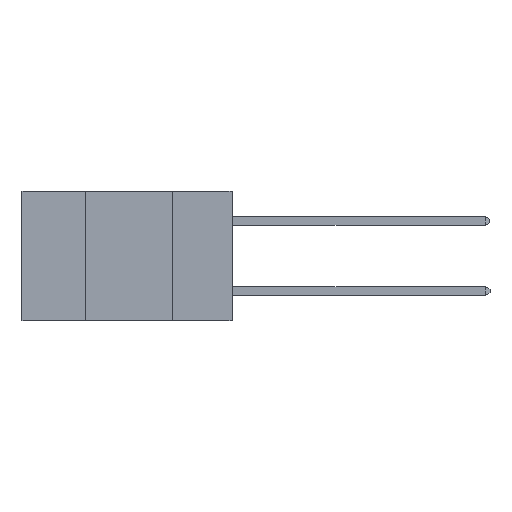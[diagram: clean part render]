
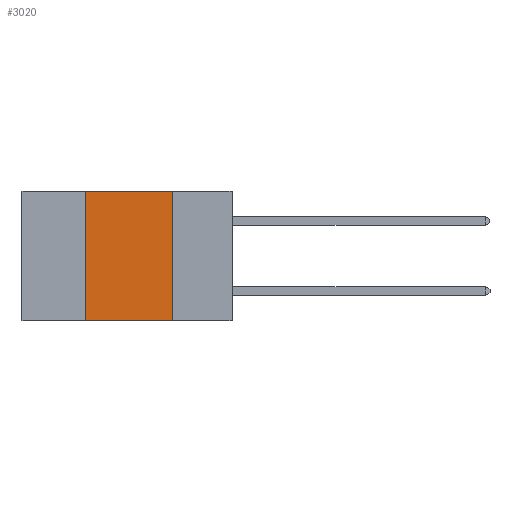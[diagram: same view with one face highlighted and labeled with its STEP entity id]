
A CAD part, left-side view. The second image highlights one B-rep face of the part: STEP entity #3020.
In plain terms, the highlighted planar face has unit normal (-1, 0, 0).
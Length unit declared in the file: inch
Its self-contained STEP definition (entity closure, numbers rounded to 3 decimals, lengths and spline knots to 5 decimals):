
#36 = DIRECTION ( 'NONE',  ( 0., 0., 1. ) ) ;
#535 = ORIENTED_EDGE ( 'NONE', *, *, #21043, .T. ) ;
#1192 = EDGE_LOOP ( 'NONE', ( #10119, #15571, #13648, #535 ) ) ;
#1618 = VECTOR ( 'NONE', #36, 39.37008 ) ;
#2064 = DIRECTION ( 'NONE',  ( 0., -1., 0. ) ) ;
#2441 = DIRECTION ( 'NONE',  ( 0., -1., 0. ) ) ;
#2514 = CARTESIAN_POINT ( 'NONE',  ( 0., 0.6, 0. ) ) ;
#3020 = ADVANCED_FACE ( 'NONE', ( #11114 ), #13163, .F. ) ;
#3919 = EDGE_CURVE ( 'NONE', #20569, #15913, #10508, .T. ) ;
#4272 = DIRECTION ( 'NONE',  ( 0., 0., -1. ) ) ;
#5743 = CARTESIAN_POINT ( 'NONE',  ( 0., 0.42, 0. ) ) ;
#7264 = AXIS2_PLACEMENT_3D ( 'NONE', #20250, #14940, #4272 ) ;
#7804 = CARTESIAN_POINT ( 'NONE',  ( 0., 0.42, -0.37 ) ) ;
#8982 = DIRECTION ( 'NONE',  ( 0., 0., -1. ) ) ;
#9152 = VECTOR ( 'NONE', #2441, 39.37008 ) ;
#9858 = EDGE_CURVE ( 'NONE', #23024, #17463, #12923, .T. ) ;
#10119 = ORIENTED_EDGE ( 'NONE', *, *, #9858, .F. ) ;
#10508 = LINE ( 'NONE', #12519, #1618 ) ;
#10911 = CARTESIAN_POINT ( 'NONE',  ( 0., 0.6, -0.37 ) ) ;
#11114 = FACE_OUTER_BOUND ( 'NONE', #1192, .T. ) ;
#12519 = CARTESIAN_POINT ( 'NONE',  ( 0., 0.42, 0. ) ) ;
#12758 = EDGE_CURVE ( 'NONE', #15913, #23024, #13920, .T. ) ;
#12923 = LINE ( 'NONE', #17884, #17050 ) ;
#13163 = PLANE ( 'NONE',  #7264 ) ;
#13324 = CARTESIAN_POINT ( 'NONE',  ( 0., 0.17, -0.37 ) ) ;
#13648 = ORIENTED_EDGE ( 'NONE', *, *, #3919, .F. ) ;
#13920 = LINE ( 'NONE', #2514, #9152 ) ;
#14940 = DIRECTION ( 'NONE',  ( 1., 0., 0. ) ) ;
#15571 = ORIENTED_EDGE ( 'NONE', *, *, #12758, .F. ) ;
#15913 = VERTEX_POINT ( 'NONE', #5743 ) ;
#17050 = VECTOR ( 'NONE', #8982, 39.37008 ) ;
#17463 = VERTEX_POINT ( 'NONE', #13324 ) ;
#17884 = CARTESIAN_POINT ( 'NONE',  ( 0., 0.17, 0. ) ) ;
#20250 = CARTESIAN_POINT ( 'NONE',  ( 0., 0.6, 0. ) ) ;
#20569 = VERTEX_POINT ( 'NONE', #7804 ) ;
#20769 = VECTOR ( 'NONE', #2064, 39.37008 ) ;
#21043 = EDGE_CURVE ( 'NONE', #20569, #17463, #21308, .T. ) ;
#21308 = LINE ( 'NONE', #10911, #20769 ) ;
#21390 = CARTESIAN_POINT ( 'NONE',  ( 0., 0.17, 0. ) ) ;
#23024 = VERTEX_POINT ( 'NONE', #21390 ) ;
